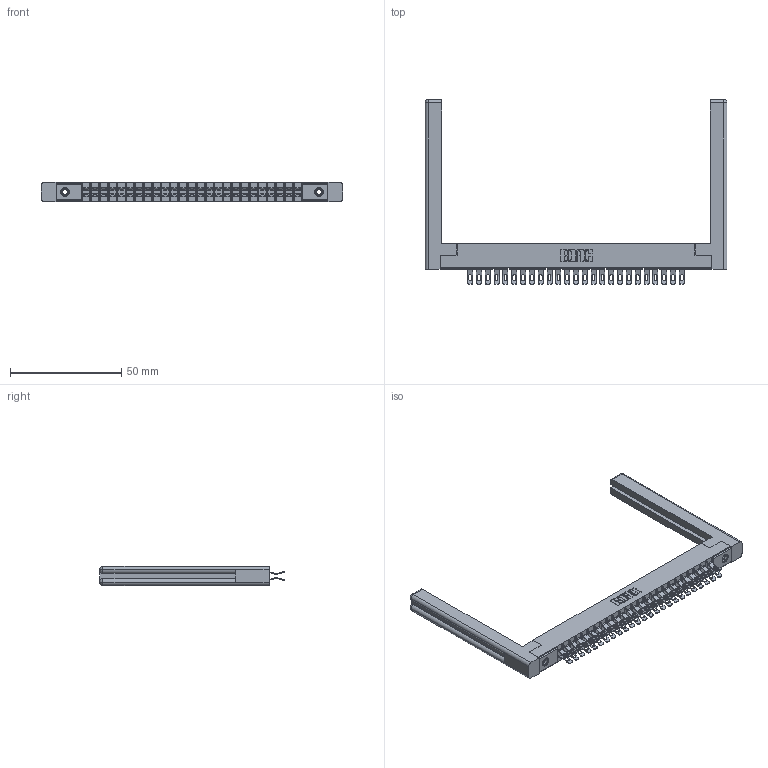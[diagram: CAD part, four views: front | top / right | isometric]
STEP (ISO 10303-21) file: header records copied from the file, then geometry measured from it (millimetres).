
FILE_DESCRIPTION (( 'STEP AP203' ), '1' );
FILE_NAME ('355-050-555-258.STEP', '2019-09-11T15:57:52', ( '' ), ( '' ), 'SwSTEP 2.0', 'SolidWorks 2016', '' );
FILE_SCHEMA (( 'CONFIG_CONTROL_DESIGN' ));
Length unit declared in the file: inch
Products named in the file (5): 305-290-001_555; 305 Part_.156 Dia; 345-250-001_345-250-001-102; 355-050-555-258; 307-220-058
Assembly tree (55 placements, depth 2):
  355-050-555-258
    305 Part_.156 Dia
    305-290-001_555  x50
    345-250-001_345-250-001-102  x2
    307-220-058  x2
Bounding box: 135.69 x 83.06 x 8.71 mm (x, y, z)
Volume: 16372.2 mm3; surface area: 22417.6 mm2
Topology: 55 solids, 55 shells, 3558 faces, 10545 edges, 6882 vertices
Faces by surface type: plane 1752, cylinder 1682, sphere 100, cone 12, torus 12
Entity records: 32395 total; most frequent: CARTESIAN_POINT 5394, ORIENTED_EDGE 5284, DIRECTION 5188, EDGE_CURVE 2642, LINE 2088, VECTOR 2088, VERTEX_POINT 1686, AXIS2_PLACEMENT_3D 1550
